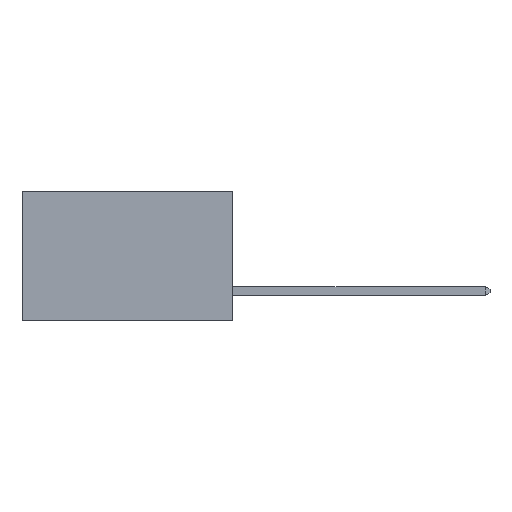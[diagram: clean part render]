
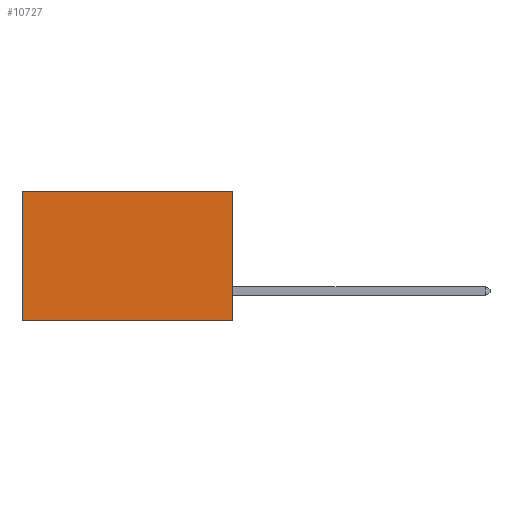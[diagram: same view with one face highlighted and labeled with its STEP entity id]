
A CAD part, left-side view. The second image highlights one B-rep face of the part: STEP entity #10727.
In plain terms, the highlighted planar face has unit normal (-1, 0, 0).
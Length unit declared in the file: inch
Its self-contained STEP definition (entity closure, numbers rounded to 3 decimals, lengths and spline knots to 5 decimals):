
#689 = EDGE_CURVE ( 'NONE', #16967, #5347, #13762, .T. ) ;
#746 = EDGE_CURVE ( 'NONE', #5347, #5056, #8446, .T. ) ;
#760 = ORIENTED_EDGE ( 'NONE', *, *, #746, .F. ) ;
#1496 = FACE_OUTER_BOUND ( 'NONE', #5209, .T. ) ;
#1828 = EDGE_CURVE ( 'NONE', #16967, #13071, #7727, .T. ) ;
#3655 = ORIENTED_EDGE ( 'NONE', *, *, #3739, .T. ) ;
#3739 = EDGE_CURVE ( 'NONE', #13071, #5056, #10892, .T. ) ;
#4650 = ORIENTED_EDGE ( 'NONE', *, *, #1828, .T. ) ;
#5056 = VERTEX_POINT ( 'NONE', #9090 ) ;
#5209 = EDGE_LOOP ( 'NONE', ( #3655, #760, #8625, #4650 ) ) ;
#5347 = VERTEX_POINT ( 'NONE', #10887 ) ;
#6274 = DIRECTION ( 'NONE',  ( 0., 0., -1. ) ) ;
#7727 = LINE ( 'NONE', #11113, #11010 ) ;
#7873 = CARTESIAN_POINT ( 'NONE',  ( 0.2875, 0., 0. ) ) ;
#8446 = LINE ( 'NONE', #14644, #15233 ) ;
#8625 = ORIENTED_EDGE ( 'NONE', *, *, #689, .F. ) ;
#9090 = CARTESIAN_POINT ( 'NONE',  ( 0.2875, 0.6, -0.37 ) ) ;
#9305 = DIRECTION ( 'NONE',  ( 0., 0., -1. ) ) ;
#10135 = CARTESIAN_POINT ( 'NONE',  ( 0.2875, 0.6, 0. ) ) ;
#10480 = DIRECTION ( 'NONE',  ( 0., 0., -1. ) ) ;
#10727 = ADVANCED_FACE ( 'NONE', ( #1496 ), #14656, .F. ) ;
#10887 = CARTESIAN_POINT ( 'NONE',  ( 0.2875, 0., -0.37 ) ) ;
#10892 = LINE ( 'NONE', #10135, #14027 ) ;
#11010 = VECTOR ( 'NONE', #17734, 39.37008 ) ;
#11113 = CARTESIAN_POINT ( 'NONE',  ( 0.2875, 0., 0. ) ) ;
#13071 = VERTEX_POINT ( 'NONE', #17830 ) ;
#13342 = VECTOR ( 'NONE', #6274, 39.37008 ) ;
#13762 = LINE ( 'NONE', #17152, #13342 ) ;
#14027 = VECTOR ( 'NONE', #10480, 39.37008 ) ;
#14644 = CARTESIAN_POINT ( 'NONE',  ( 0.2875, 0., -0.37 ) ) ;
#14656 = PLANE ( 'NONE',  #15070 ) ;
#15070 = AXIS2_PLACEMENT_3D ( 'NONE', #7873, #17334, #9305 ) ;
#15233 = VECTOR ( 'NONE', #17377, 39.37008 ) ;
#15275 = CARTESIAN_POINT ( 'NONE',  ( 0.2875, 0., 0. ) ) ;
#16967 = VERTEX_POINT ( 'NONE', #15275 ) ;
#17152 = CARTESIAN_POINT ( 'NONE',  ( 0.2875, 0., 0. ) ) ;
#17334 = DIRECTION ( 'NONE',  ( 1., 0., 0. ) ) ;
#17377 = DIRECTION ( 'NONE',  ( 0., 1., 0. ) ) ;
#17734 = DIRECTION ( 'NONE',  ( 0., 1., 0. ) ) ;
#17830 = CARTESIAN_POINT ( 'NONE',  ( 0.2875, 0.6, 0. ) ) ;
